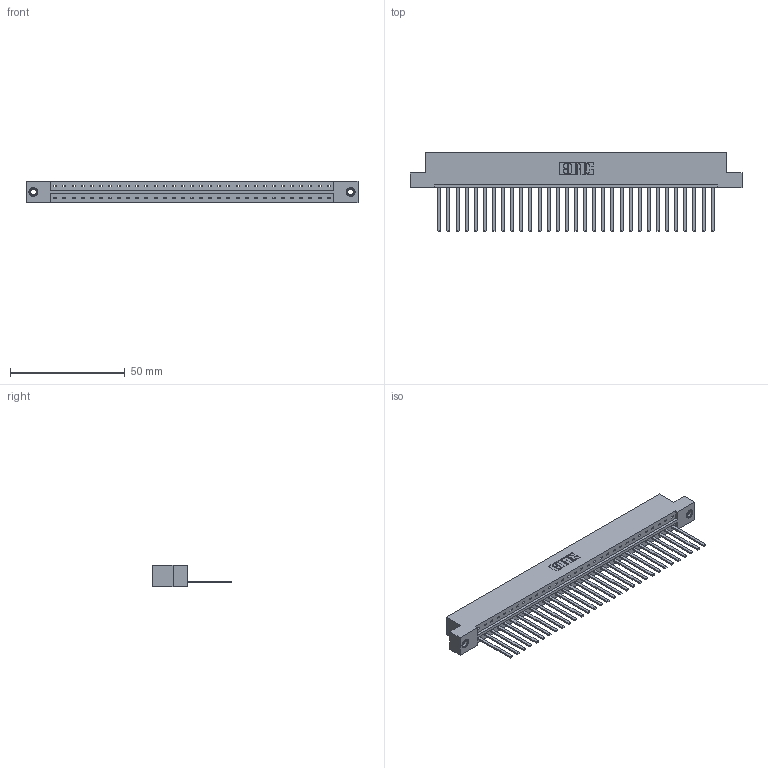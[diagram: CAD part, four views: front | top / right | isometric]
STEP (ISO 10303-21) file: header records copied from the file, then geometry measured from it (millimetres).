
FILE_DESCRIPTION (( 'STEP AP203' ), '1' );
FILE_NAME ('833-031-544-107.STEP', '2020-06-02T15:52:54', ( '' ), ( '' ), 'SwSTEP 2.0', 'SolidWorks 2020', '' );
FILE_SCHEMA (( 'CONFIG_CONTROL_DESIGN' ));
Length unit declared in the file: inch
Products named in the file (4): 345-250-001_345-250-005-103; 833-031-544-107; 345-292-001_345-293-144; 833 Part_Flush - .156 Dia - TI
Assembly tree (34 placements, depth 2):
  833-031-544-107
    833 Part_Flush - .156 Dia - TI
    345-292-001_345-293-144  x31
    345-250-001_345-250-005-103  x2
Bounding box: 144.37 x 34.3 x 9.4 mm (x, y, z)
Volume: 14779 mm3; surface area: 17123.5 mm2
Topology: 34 solids, 34 shells, 1786 faces, 5345 edges, 3514 vertices
Faces by surface type: plane 1280, cylinder 490, cone 12, torus 4
Entity records: 21376 total; most frequent: CARTESIAN_POINT 3670, ORIENTED_EDGE 3630, DIRECTION 3147, EDGE_CURVE 1815, VECTOR 1671, LINE 1671, VERTEX_POINT 1204, AXIS2_PLACEMENT_3D 738
